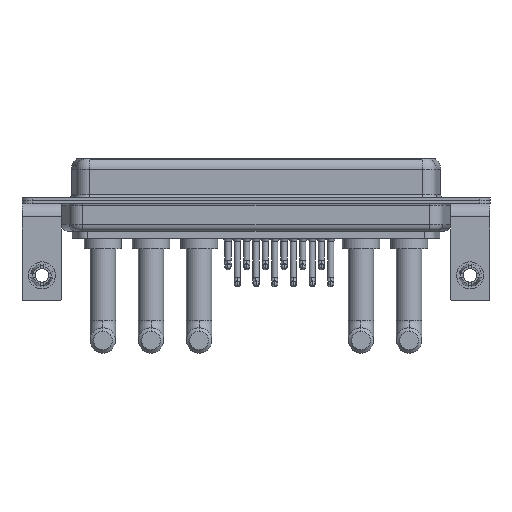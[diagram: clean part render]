
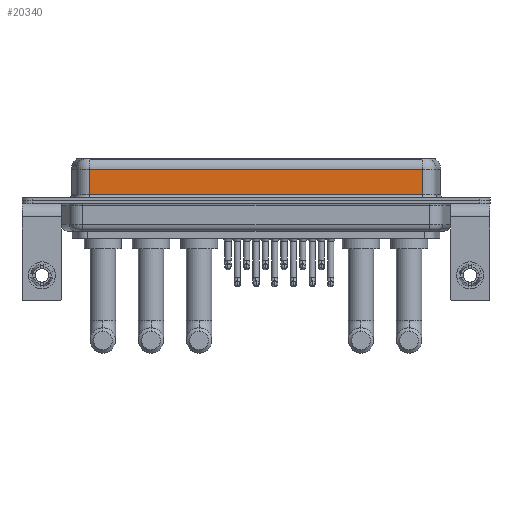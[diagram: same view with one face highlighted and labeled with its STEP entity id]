
A CAD part, front view. The second image highlights one B-rep face of the part: STEP entity #20340.
In plain terms, the highlighted planar face has unit normal (0, -1, 0).
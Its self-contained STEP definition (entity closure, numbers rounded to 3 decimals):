
#17 = AXIS2_PLACEMENT_3D ( 'NONE', #11369, #18677, #11604 ) ;
#26 = VECTOR ( 'NONE', #3000, 1000. ) ;
#2790 = LINE ( 'NONE', #6235, #11903 ) ;
#2857 = PLANE ( 'NONE',  #17 ) ;
#3000 = DIRECTION ( 'NONE',  ( 0., 0., -1. ) ) ;
#3289 = ORIENTED_EDGE ( 'NONE', *, *, #3914, .T. ) ;
#3303 = DIRECTION ( 'NONE',  ( 0., 0., -1. ) ) ;
#3914 = EDGE_CURVE ( 'NONE', #9905, #13544, #4834, .T. ) ;
#4693 = FACE_OUTER_BOUND ( 'NONE', #16996, .T. ) ;
#4799 = LINE ( 'NONE', #11597, #13166 ) ;
#4834 = LINE ( 'NONE', #10229, #26 ) ;
#6235 = CARTESIAN_POINT ( 'NONE',  ( 56.462, -3.95, 4.65 ) ) ;
#6614 = ORIENTED_EDGE ( 'NONE', *, *, #10953, .T. ) ;
#6848 = VECTOR ( 'NONE', #12041, 1000. ) ;
#8871 = ORIENTED_EDGE ( 'NONE', *, *, #13511, .T. ) ;
#9650 = CARTESIAN_POINT ( 'NONE',  ( 56.462, -3.95, 0.9 ) ) ;
#9905 = VERTEX_POINT ( 'NONE', #16312 ) ;
#10229 = CARTESIAN_POINT ( 'NONE',  ( 7.038, -3.95, 6.4 ) ) ;
#10311 = LINE ( 'NONE', #15704, #6848 ) ;
#10953 = EDGE_CURVE ( 'NONE', #14060, #9905, #2790, .T. ) ;
#11356 = VERTEX_POINT ( 'NONE', #9650 ) ;
#11369 = CARTESIAN_POINT ( 'NONE',  ( 56.462, -3.95, 6.4 ) ) ;
#11597 = CARTESIAN_POINT ( 'NONE',  ( 56.462, -3.95, 6.4 ) ) ;
#11604 = DIRECTION ( 'NONE',  ( 0., 0., 1. ) ) ;
#11903 = VECTOR ( 'NONE', #22024, 1000. ) ;
#12041 = DIRECTION ( 'NONE',  ( 1., 0., 0. ) ) ;
#13166 = VECTOR ( 'NONE', #3303, 1000. ) ;
#13511 = EDGE_CURVE ( 'NONE', #13544, #11356, #10311, .T. ) ;
#13544 = VERTEX_POINT ( 'NONE', #18996 ) ;
#14060 = VERTEX_POINT ( 'NONE', #17426 ) ;
#15704 = CARTESIAN_POINT ( 'NONE',  ( 56.462, -3.95, 0.9 ) ) ;
#16312 = CARTESIAN_POINT ( 'NONE',  ( 7.038, -3.95, 4.65 ) ) ;
#16996 = EDGE_LOOP ( 'NONE', ( #21345, #6614, #3289, #8871 ) ) ;
#17158 = EDGE_CURVE ( 'NONE', #14060, #11356, #4799, .T. ) ;
#17426 = CARTESIAN_POINT ( 'NONE',  ( 56.462, -3.95, 4.65 ) ) ;
#18677 = DIRECTION ( 'NONE',  ( 0., 1., 0. ) ) ;
#18996 = CARTESIAN_POINT ( 'NONE',  ( 7.038, -3.95, 0.9 ) ) ;
#20340 = ADVANCED_FACE ( 'NONE', ( #4693 ), #2857, .F. ) ;
#21345 = ORIENTED_EDGE ( 'NONE', *, *, #17158, .F. ) ;
#22024 = DIRECTION ( 'NONE',  ( -1., 0., 0. ) ) ;
